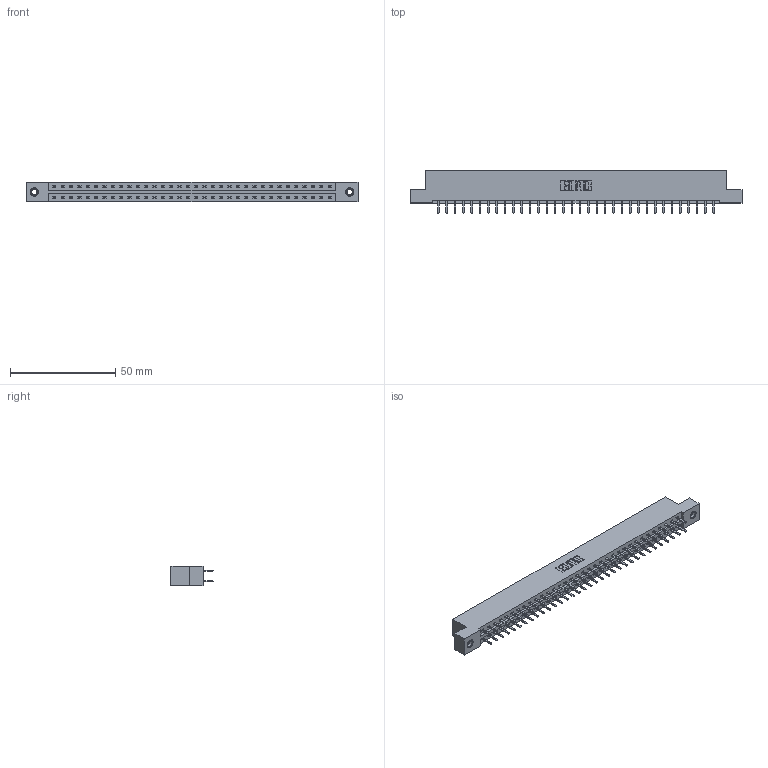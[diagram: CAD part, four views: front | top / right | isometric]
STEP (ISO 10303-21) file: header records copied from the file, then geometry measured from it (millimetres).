
FILE_DESCRIPTION (( 'STEP AP203' ), '1' );
FILE_NAME ('387-068-520-207.STEP', '2018-09-21T11:58:41', ( '' ), ( '' ), 'SwSTEP 2.0', 'SolidWorks 2016', '' );
FILE_SCHEMA (( 'CONFIG_CONTROL_DESIGN' ));
Length unit declared in the file: inch
Products named in the file (4): 345-292-001_345-293-120; 345-250-001_345-250-005-103; 387-068-520-207; 337 Part_Flush Mounting Lugs - 0.156 Dia-TI
Assembly tree (71 placements, depth 2):
  387-068-520-207
    337 Part_Flush Mounting Lugs - 0.156 Dia-TI
    345-292-001_345-293-120  x68
    345-250-001_345-250-005-103  x2
Bounding box: 157.73 x 20.02 x 9.4 mm (x, y, z)
Volume: 16473.4 mm3; surface area: 18496.1 mm2
Topology: 71 solids, 71 shells, 4118 faces, 11939 edges, 7770 vertices
Faces by surface type: plane 2822, cylinder 1280, cone 12, torus 4
Entity records: 28696 total; most frequent: CARTESIAN_POINT 4833, ORIENTED_EDGE 4750, DIRECTION 4145, EDGE_CURVE 2375, LINE 2223, VECTOR 2223, VERTEX_POINT 1576, AXIS2_PLACEMENT_3D 961
